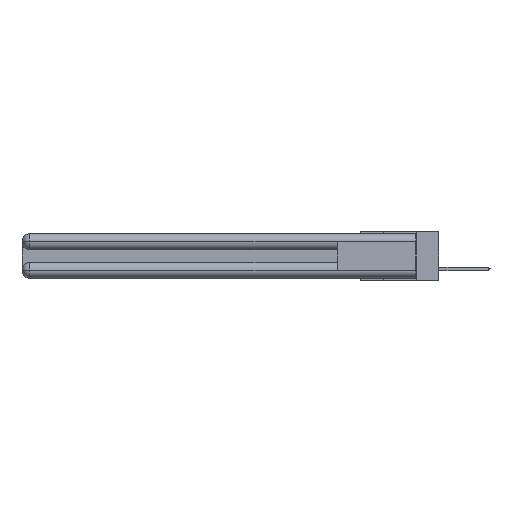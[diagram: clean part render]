
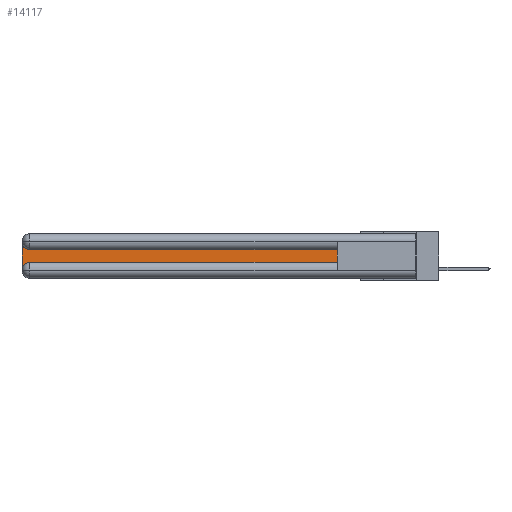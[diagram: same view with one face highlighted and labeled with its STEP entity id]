
A CAD part, left-side view. The second image highlights one B-rep face of the part: STEP entity #14117.
In plain terms, the highlighted planar face has unit normal (-1, 0, 0).
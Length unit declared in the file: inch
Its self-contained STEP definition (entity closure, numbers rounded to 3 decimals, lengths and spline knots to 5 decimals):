
#1034 = VERTEX_POINT ( 'NONE', #5103 ) ;
#1685 = DIRECTION ( 'NONE',  ( 0., 0., -1. ) ) ;
#1958 = VECTOR ( 'NONE', #6406, 39.37008 ) ;
#2409 = LINE ( 'NONE', #25651, #24649 ) ;
#2624 = CARTESIAN_POINT ( 'NONE',  ( 0.075, 0.6, -0.2175 ) ) ;
#2906 = EDGE_CURVE ( 'NONE', #1034, #26213, #13383, .T. ) ;
#3726 = CARTESIAN_POINT ( 'NONE',  ( 0.075, 3., -0.2175 ) ) ;
#3896 = CIRCLE ( 'NONE', #11175, 0.06 ) ;
#4003 = DIRECTION ( 'NONE',  ( 0., 0., -1. ) ) ;
#4345 = VERTEX_POINT ( 'NONE', #2624 ) ;
#4509 = DIRECTION ( 'NONE',  ( 1., 0., 0. ) ) ;
#5103 = CARTESIAN_POINT ( 'NONE',  ( 0.075, 0.6, -0.1225 ) ) ;
#5773 = AXIS2_PLACEMENT_3D ( 'NONE', #23835, #4509, #19876 ) ;
#5903 = ORIENTED_EDGE ( 'NONE', *, *, #17343, .T. ) ;
#5950 = FACE_OUTER_BOUND ( 'NONE', #27541, .T. ) ;
#6361 = EDGE_CURVE ( 'NONE', #26435, #4345, #10357, .T. ) ;
#6406 = DIRECTION ( 'NONE',  ( 0., 1., 0. ) ) ;
#8338 = CARTESIAN_POINT ( 'NONE',  ( 0.075, 2.94, -0.0625 ) ) ;
#8814 = EDGE_CURVE ( 'NONE', #4345, #1034, #2409, .T. ) ;
#10357 = LINE ( 'NONE', #26524, #19819 ) ;
#10434 = CARTESIAN_POINT ( 'NONE',  ( 0.075, 0.6, -0.1225 ) ) ;
#10758 = DIRECTION ( 'NONE',  ( 0., 0., 1. ) ) ;
#11175 = AXIS2_PLACEMENT_3D ( 'NONE', #8338, #27625, #4003 ) ;
#12030 = ORIENTED_EDGE ( 'NONE', *, *, #6361, .T. ) ;
#13383 = LINE ( 'NONE', #10434, #1958 ) ;
#13880 = CIRCLE ( 'NONE', #5773, 0.06 ) ;
#13926 = VERTEX_POINT ( 'NONE', #22577 ) ;
#14117 = ADVANCED_FACE ( 'NONE', ( #5950 ), #27272, .F. ) ;
#16612 = DIRECTION ( 'NONE',  ( 1., 0., 0. ) ) ;
#16712 = CARTESIAN_POINT ( 'NONE',  ( 0.075, 3., -0.1225 ) ) ;
#17343 = EDGE_CURVE ( 'NONE', #13926, #19224, #23032, .T. ) ;
#17643 = DIRECTION ( 'NONE',  ( 0., -1., 0. ) ) ;
#18304 = VECTOR ( 'NONE', #1685, 39.37008 ) ;
#18884 = ORIENTED_EDGE ( 'NONE', *, *, #8814, .T. ) ;
#18992 = DIRECTION ( 'NONE',  ( 0., 0., -1. ) ) ;
#19224 = VERTEX_POINT ( 'NONE', #21612 ) ;
#19819 = VECTOR ( 'NONE', #17643, 39.37008 ) ;
#19876 = DIRECTION ( 'NONE',  ( 0., 0., -1. ) ) ;
#20229 = EDGE_CURVE ( 'NONE', #26213, #13926, #3896, .T. ) ;
#21590 = EDGE_CURVE ( 'NONE', #19224, #26435, #13880, .T. ) ;
#21610 = CARTESIAN_POINT ( 'NONE',  ( 0.075, 2.94, -0.2175 ) ) ;
#21612 = CARTESIAN_POINT ( 'NONE',  ( 0.075, 3., -0.2775 ) ) ;
#22577 = CARTESIAN_POINT ( 'NONE',  ( 0.075, 3., -0.0625 ) ) ;
#22866 = ORIENTED_EDGE ( 'NONE', *, *, #21590, .T. ) ;
#23032 = LINE ( 'NONE', #3726, #18304 ) ;
#23483 = ORIENTED_EDGE ( 'NONE', *, *, #20229, .T. ) ;
#23835 = CARTESIAN_POINT ( 'NONE',  ( 0.075, 2.94, -0.2775 ) ) ;
#23901 = AXIS2_PLACEMENT_3D ( 'NONE', #16712, #16612, #18992 ) ;
#24649 = VECTOR ( 'NONE', #10758, 39.37008 ) ;
#25651 = CARTESIAN_POINT ( 'NONE',  ( 0.075, 0.6, -0.2175 ) ) ;
#26213 = VERTEX_POINT ( 'NONE', #27261 ) ;
#26435 = VERTEX_POINT ( 'NONE', #21610 ) ;
#26524 = CARTESIAN_POINT ( 'NONE',  ( 0.075, 0.6, -0.2175 ) ) ;
#27261 = CARTESIAN_POINT ( 'NONE',  ( 0.075, 2.94, -0.1225 ) ) ;
#27272 = PLANE ( 'NONE',  #23901 ) ;
#27441 = ORIENTED_EDGE ( 'NONE', *, *, #2906, .T. ) ;
#27541 = EDGE_LOOP ( 'NONE', ( #27441, #23483, #5903, #22866, #12030, #18884 ) ) ;
#27625 = DIRECTION ( 'NONE',  ( 1., 0., 0. ) ) ;
